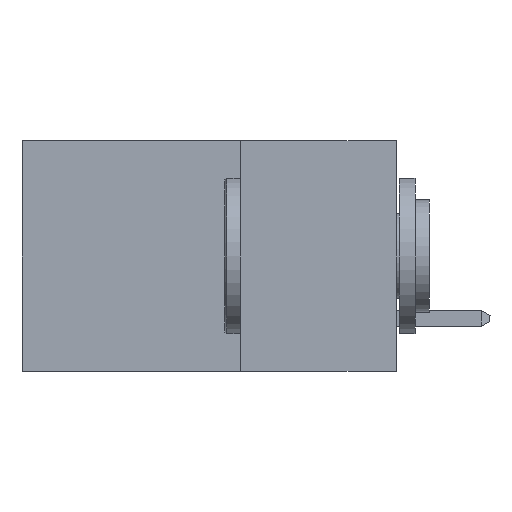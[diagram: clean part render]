
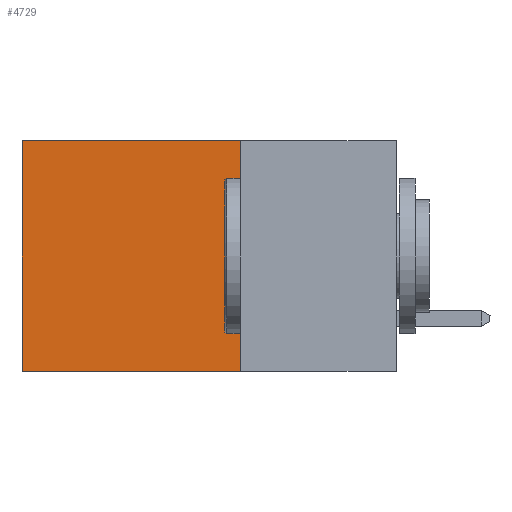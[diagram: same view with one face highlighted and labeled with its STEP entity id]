
A CAD part, left-side view. The second image highlights one B-rep face of the part: STEP entity #4729.
In plain terms, the highlighted planar face has unit normal (-1, 0, 0).
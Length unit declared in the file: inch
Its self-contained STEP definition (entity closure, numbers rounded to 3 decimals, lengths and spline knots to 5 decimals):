
#378 = LINE ( 'NONE', #3746, #1309 ) ;
#914 = EDGE_CURVE ( 'NONE', #3653, #6910, #8419, .T. ) ;
#984 = CARTESIAN_POINT ( 'NONE',  ( 0.2615, 0.25, -0.37 ) ) ;
#1309 = VECTOR ( 'NONE', #10505, 39.37008 ) ;
#1395 = CARTESIAN_POINT ( 'NONE',  ( 0.2615, 0.6, -0.37 ) ) ;
#1485 = DIRECTION ( 'NONE',  ( 0., 0., -1. ) ) ;
#1558 = LINE ( 'NONE', #10030, #3578 ) ;
#1656 = DIRECTION ( 'NONE',  ( 0., 1., 0. ) ) ;
#1694 = ORIENTED_EDGE ( 'NONE', *, *, #9572, .F. ) ;
#2195 = LINE ( 'NONE', #5741, #2648 ) ;
#2380 = CARTESIAN_POINT ( 'NONE',  ( 0.2615, 0.25, 0. ) ) ;
#2610 = CARTESIAN_POINT ( 'NONE',  ( 0.2615, 0.6, 0. ) ) ;
#2648 = VECTOR ( 'NONE', #1485, 39.37008 ) ;
#3578 = VECTOR ( 'NONE', #9144, 39.37008 ) ;
#3653 = VERTEX_POINT ( 'NONE', #9936 ) ;
#3746 = CARTESIAN_POINT ( 'NONE',  ( 0.2615, 0.25, -0.37 ) ) ;
#4162 = VERTEX_POINT ( 'NONE', #1395 ) ;
#4347 = DIRECTION ( 'NONE',  ( 0., 0., -1. ) ) ;
#4606 = EDGE_CURVE ( 'NONE', #6910, #4162, #2195, .T. ) ;
#4729 = ADVANCED_FACE ( 'NONE', ( #6674 ), #8569, .F. ) ;
#5667 = CARTESIAN_POINT ( 'NONE',  ( 0.2615, 0.25, -0.37 ) ) ;
#5741 = CARTESIAN_POINT ( 'NONE',  ( 0.2615, 0.6, -0.37 ) ) ;
#5999 = AXIS2_PLACEMENT_3D ( 'NONE', #984, #7734, #4347 ) ;
#6674 = FACE_OUTER_BOUND ( 'NONE', #8676, .T. ) ;
#6838 = VECTOR ( 'NONE', #1656, 39.37008 ) ;
#6910 = VERTEX_POINT ( 'NONE', #2610 ) ;
#7377 = ORIENTED_EDGE ( 'NONE', *, *, #8581, .F. ) ;
#7734 = DIRECTION ( 'NONE',  ( 1., 0., 0. ) ) ;
#8299 = ORIENTED_EDGE ( 'NONE', *, *, #4606, .T. ) ;
#8419 = LINE ( 'NONE', #2380, #6838 ) ;
#8569 = PLANE ( 'NONE',  #5999 ) ;
#8581 = EDGE_CURVE ( 'NONE', #10850, #4162, #378, .T. ) ;
#8676 = EDGE_LOOP ( 'NONE', ( #8299, #7377, #1694, #10278 ) ) ;
#9144 = DIRECTION ( 'NONE',  ( 0., 0., -1. ) ) ;
#9572 = EDGE_CURVE ( 'NONE', #3653, #10850, #1558, .T. ) ;
#9936 = CARTESIAN_POINT ( 'NONE',  ( 0.2615, 0.25, 0. ) ) ;
#10030 = CARTESIAN_POINT ( 'NONE',  ( 0.2615, 0.25, -0.37 ) ) ;
#10278 = ORIENTED_EDGE ( 'NONE', *, *, #914, .T. ) ;
#10505 = DIRECTION ( 'NONE',  ( 0., 1., 0. ) ) ;
#10850 = VERTEX_POINT ( 'NONE', #5667 ) ;
